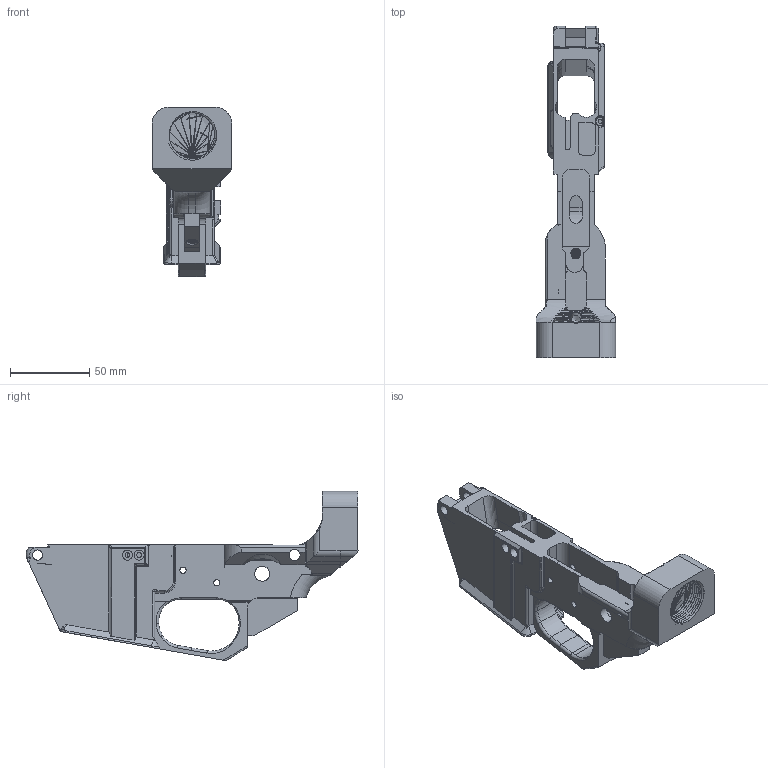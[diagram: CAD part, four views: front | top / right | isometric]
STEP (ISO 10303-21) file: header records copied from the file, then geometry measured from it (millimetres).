
FILE_DESCRIPTION(/* description */ (''),/* implementation_level */ '2;1');
FILE_NAME(/* name */ 'ar9.step',/* time_stamp */ '2019-07-15T13:09:14-04:00',/* author */ (''),/* organization */ (''),/* preprocessor_version */ 'ST-DEVELOPER v18',/* originating_system */ 'Autodesk Translation Framework v8.2.0.1029',/* authorisation */ '');
FILE_SCHEMA (('AUTOMOTIVE_DESIGN { 1 0 10303 214 3 1 1 }'));
Products named in the file (1): ar9
Bounding box: 50.01 x 209.05 x 106.55 mm (x, y, z)
Volume: 171561.4 mm3; surface area: 60008.3 mm2
Topology: 1 solids, 1 shells, 769 faces, 2250 edges, 1467 vertices
Faces by surface type: cylinder 321, plane 237, bspline 137, torus 47, cone 16, sphere 11
Full cylindrical faces by diameter (mm): 1.934 x1, 2.464 x1, 2.529 x20, 2.54 x1, 3 x4, 3.086 x4, 3.175 x1, 3.962 x4, 5.172 x21, 6.35 x21, 6.352 x2, 6.375 x2, 6.477 x1, 7 x2, 7.925 x1, 9.525 x2, 28.575 x13
Entity records: 79696 total; most frequent: CARTESIAN_POINT 60533, ORIENTED_EDGE 4476, DIRECTION 3428, EDGE_CURVE 2238, VERTEX_POINT 1467, AXIS2_PLACEMENT_3D 1269, LINE 890, VECTOR 890
